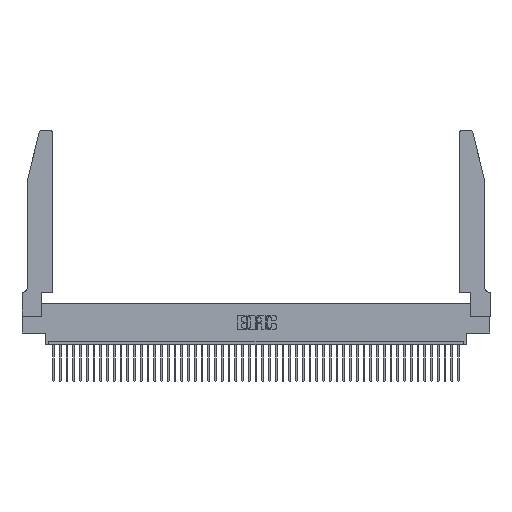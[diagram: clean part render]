
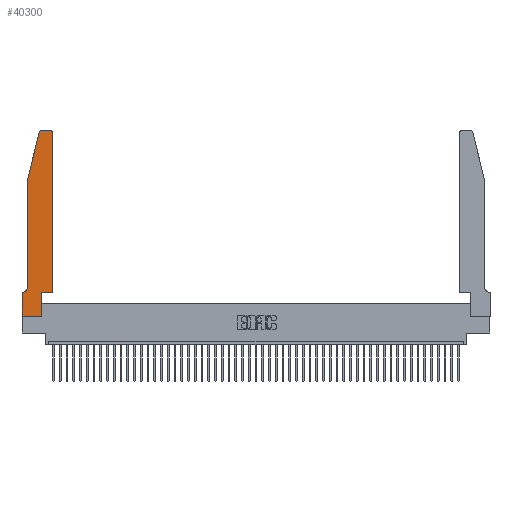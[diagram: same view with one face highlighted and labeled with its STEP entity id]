
A CAD part, top view. The second image highlights one B-rep face of the part: STEP entity #40300.
In plain terms, the highlighted planar face has unit normal (0, 0, 1).
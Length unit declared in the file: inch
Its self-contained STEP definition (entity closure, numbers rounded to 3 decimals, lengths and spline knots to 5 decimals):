
#464 = ORIENTED_EDGE ( 'NONE', *, *, #37919, .T. ) ;
#1316 = CARTESIAN_POINT ( 'NONE',  ( 0.25487, 2.72718, 0.37 ) ) ;
#1873 = EDGE_CURVE ( 'NONE', #12981, #21271, #39170, .T. ) ;
#2522 = PLANE ( 'NONE',  #16732 ) ;
#2717 = CARTESIAN_POINT ( 'NONE',  ( 0.4205, 2.72, 0.37 ) ) ;
#4221 = CARTESIAN_POINT ( 'NONE',  ( 0.0755, 2., 0.37 ) ) ;
#4339 = ORIENTED_EDGE ( 'NONE', *, *, #26272, .T. ) ;
#4389 = CARTESIAN_POINT ( 'NONE',  ( 0.284, 2.75, 0.37 ) ) ;
#5014 = CARTESIAN_POINT ( 'NONE',  ( 0.0055, 0.35, 0.37 ) ) ;
#6638 = ORIENTED_EDGE ( 'NONE', *, *, #16581, .T. ) ;
#7432 = EDGE_CURVE ( 'NONE', #38609, #40863, #31435, .T. ) ;
#9850 = EDGE_CURVE ( 'NONE', #31386, #45186, #26042, .T. ) ;
#10083 = ORIENTED_EDGE ( 'NONE', *, *, #23843, .T. ) ;
#12249 = ORIENTED_EDGE ( 'NONE', *, *, #21033, .T. ) ;
#12276 = CARTESIAN_POINT ( 'NONE',  ( 0.0055, 0.42, 0.37 ) ) ;
#12981 = VERTEX_POINT ( 'NONE', #15764 ) ;
#13245 = FACE_OUTER_BOUND ( 'NONE', #35710, .T. ) ;
#13918 = VERTEX_POINT ( 'NONE', #27395 ) ;
#13920 = LINE ( 'NONE', #4221, #45905 ) ;
#14765 = CARTESIAN_POINT ( 'NONE',  ( 0., 0., 0.37 ) ) ;
#15764 = CARTESIAN_POINT ( 'NONE',  ( 0.0755, 0.42, 0.37 ) ) ;
#16581 = EDGE_CURVE ( 'NONE', #21271, #37351, #20579, .T. ) ;
#16732 = AXIS2_PLACEMENT_3D ( 'NONE', #39683, #43271, #25166 ) ;
#17110 = DIRECTION ( 'NONE',  ( 0., 1., 0. ) ) ;
#17437 = CARTESIAN_POINT ( 'NONE',  ( 0.4505, 0.35, 0.37 ) ) ;
#17937 = CARTESIAN_POINT ( 'NONE',  ( 0.4505, 2.72, 0.37 ) ) ;
#18596 = DIRECTION ( 'NONE',  ( 1., 0., 0. ) ) ;
#19495 = CARTESIAN_POINT ( 'NONE',  ( 0., 0., 0.37 ) ) ;
#19608 = DIRECTION ( 'NONE',  ( -1., 0., 0. ) ) ;
#19822 = VERTEX_POINT ( 'NONE', #30191 ) ;
#20154 = VECTOR ( 'NONE', #44855, 39.37008 ) ;
#20377 = LINE ( 'NONE', #41787, #29166 ) ;
#20579 = LINE ( 'NONE', #25018, #24646 ) ;
#21033 = EDGE_CURVE ( 'NONE', #40863, #13918, #45414, .T. ) ;
#21089 = CARTESIAN_POINT ( 'NONE',  ( 0.2865, 0., 0.37 ) ) ;
#21271 = VERTEX_POINT ( 'NONE', #5014 ) ;
#22914 = DIRECTION ( 'NONE',  ( 0., -1., 0. ) ) ;
#23102 = VECTOR ( 'NONE', #25284, 39.37008 ) ;
#23843 = EDGE_CURVE ( 'NONE', #19822, #28981, #30059, .T. ) ;
#23888 = ORIENTED_EDGE ( 'NONE', *, *, #1873, .T. ) ;
#24646 = VECTOR ( 'NONE', #35460, 39.37008 ) ;
#25018 = CARTESIAN_POINT ( 'NONE',  ( 0.0755, 0.35, 0.37 ) ) ;
#25128 = CARTESIAN_POINT ( 'NONE',  ( 0.0755, 2., 0.37 ) ) ;
#25166 = DIRECTION ( 'NONE',  ( 1., 0., 0. ) ) ;
#25284 = DIRECTION ( 'NONE',  ( -0.239, -0.971, 0. ) ) ;
#25635 = VECTOR ( 'NONE', #25709, 39.37008 ) ;
#25709 = DIRECTION ( 'NONE',  ( 0., -1., 0. ) ) ;
#26042 = LINE ( 'NONE', #25128, #23102 ) ;
#26272 = EDGE_CURVE ( 'NONE', #40465, #31386, #48090, .T. ) ;
#26458 = EDGE_CURVE ( 'NONE', #37351, #19822, #36772, .T. ) ;
#27395 = CARTESIAN_POINT ( 'NONE',  ( 0.4205, 2.75, 0.37 ) ) ;
#27788 = AXIS2_PLACEMENT_3D ( 'NONE', #12276, #45817, #42417 ) ;
#27960 = CARTESIAN_POINT ( 'NONE',  ( 0.0755, 2., 0.37 ) ) ;
#28659 = DIRECTION ( 'NONE',  ( 0., 1., 0. ) ) ;
#28981 = VERTEX_POINT ( 'NONE', #21089 ) ;
#29166 = VECTOR ( 'NONE', #19608, 39.37008 ) ;
#30059 = LINE ( 'NONE', #14765, #20154 ) ;
#30191 = CARTESIAN_POINT ( 'NONE',  ( 0., 0., 0.37 ) ) ;
#30248 = VECTOR ( 'NONE', #17110, 39.37008 ) ;
#30661 = VECTOR ( 'NONE', #18596, 39.37008 ) ;
#31386 = VERTEX_POINT ( 'NONE', #1316 ) ;
#31435 = LINE ( 'NONE', #17437, #30248 ) ;
#31877 = LINE ( 'NONE', #33451, #30661 ) ;
#32639 = DIRECTION ( 'NONE',  ( 0., 0., 1. ) ) ;
#33291 = CARTESIAN_POINT ( 'NONE',  ( 0.4505, 0.35, 0.37 ) ) ;
#33451 = CARTESIAN_POINT ( 'NONE',  ( 0.4505, 0.35, 0.37 ) ) ;
#33629 = DIRECTION ( 'NONE',  ( 1., 0., 0. ) ) ;
#33768 = CARTESIAN_POINT ( 'NONE',  ( 0., 0.35, 0.37 ) ) ;
#33769 = VERTEX_POINT ( 'NONE', #46875 ) ;
#34475 = LINE ( 'NONE', #43816, #43282 ) ;
#34716 = ORIENTED_EDGE ( 'NONE', *, *, #44654, .T. ) ;
#35460 = DIRECTION ( 'NONE',  ( -1., 0., 0. ) ) ;
#35710 = EDGE_LOOP ( 'NONE', ( #464, #4339, #45124, #34716, #23888, #6638, #38140, #10083, #40182, #47227, #36939, #12249 ) ) ;
#36412 = DIRECTION ( 'NONE',  ( 1., 0., 0. ) ) ;
#36772 = LINE ( 'NONE', #19495, #25635 ) ;
#36939 = ORIENTED_EDGE ( 'NONE', *, *, #7432, .T. ) ;
#37351 = VERTEX_POINT ( 'NONE', #33768 ) ;
#37919 = EDGE_CURVE ( 'NONE', #13918, #40465, #20377, .T. ) ;
#38140 = ORIENTED_EDGE ( 'NONE', *, *, #26458, .T. ) ;
#38609 = VERTEX_POINT ( 'NONE', #33291 ) ;
#39170 = CIRCLE ( 'NONE', #27788, 0.07 ) ;
#39469 = AXIS2_PLACEMENT_3D ( 'NONE', #39811, #32639, #36412 ) ;
#39683 = CARTESIAN_POINT ( 'NONE',  ( 0., 0.35, 0.37 ) ) ;
#39811 = CARTESIAN_POINT ( 'NONE',  ( 0.284, 2.72, 0.37 ) ) ;
#40048 = DIRECTION ( 'NONE',  ( 0., 0., 1. ) ) ;
#40182 = ORIENTED_EDGE ( 'NONE', *, *, #42707, .T. ) ;
#40300 = ADVANCED_FACE ( 'NONE', ( #13245 ), #2522, .T. ) ;
#40337 = EDGE_CURVE ( 'NONE', #33769, #38609, #31877, .T. ) ;
#40465 = VERTEX_POINT ( 'NONE', #4389 ) ;
#40546 = AXIS2_PLACEMENT_3D ( 'NONE', #2717, #40048, #33629 ) ;
#40863 = VERTEX_POINT ( 'NONE', #17937 ) ;
#41787 = CARTESIAN_POINT ( 'NONE',  ( 0.2605, 2.75, 0.37 ) ) ;
#42417 = DIRECTION ( 'NONE',  ( -1., 0., 0. ) ) ;
#42707 = EDGE_CURVE ( 'NONE', #28981, #33769, #34475, .T. ) ;
#43271 = DIRECTION ( 'NONE',  ( 0., 0., 1. ) ) ;
#43282 = VECTOR ( 'NONE', #28659, 39.37008 ) ;
#43816 = CARTESIAN_POINT ( 'NONE',  ( 0.2865, 0.35, 0.37 ) ) ;
#44654 = EDGE_CURVE ( 'NONE', #45186, #12981, #13920, .T. ) ;
#44855 = DIRECTION ( 'NONE',  ( 1., 0., 0. ) ) ;
#45124 = ORIENTED_EDGE ( 'NONE', *, *, #9850, .T. ) ;
#45186 = VERTEX_POINT ( 'NONE', #27960 ) ;
#45414 = CIRCLE ( 'NONE', #40546, 0.03 ) ;
#45817 = DIRECTION ( 'NONE',  ( 0., 0., -1. ) ) ;
#45905 = VECTOR ( 'NONE', #22914, 39.37008 ) ;
#46875 = CARTESIAN_POINT ( 'NONE',  ( 0.2865, 0.35, 0.37 ) ) ;
#47227 = ORIENTED_EDGE ( 'NONE', *, *, #40337, .T. ) ;
#48090 = CIRCLE ( 'NONE', #39469, 0.03 ) ;
